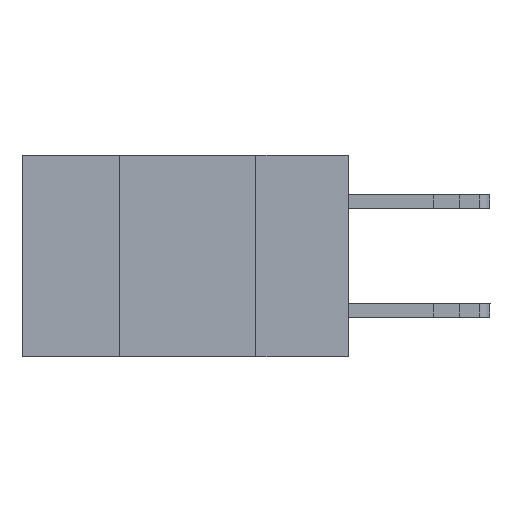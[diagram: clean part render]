
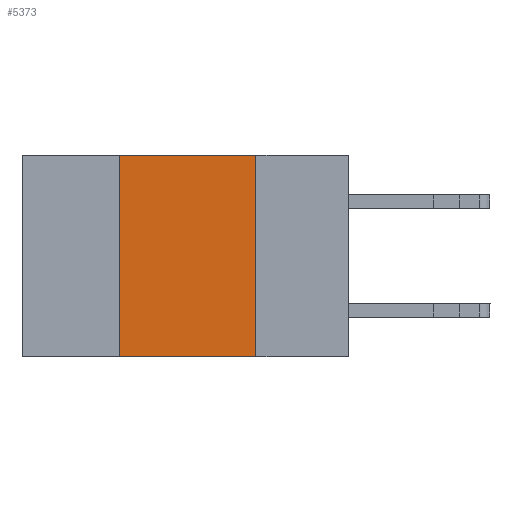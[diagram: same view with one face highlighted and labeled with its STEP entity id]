
A CAD part, left-side view. The second image highlights one B-rep face of the part: STEP entity #5373.
In plain terms, the highlighted planar face has unit normal (-1, 0, 0).
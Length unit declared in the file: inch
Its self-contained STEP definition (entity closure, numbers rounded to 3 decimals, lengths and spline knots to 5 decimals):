
#2670 = EDGE_CURVE ( 'NONE', #3437, #2915, #7472, .T. ) ;
#2915 = VERTEX_POINT ( 'NONE', #8823 ) ;
#3209 = ORIENTED_EDGE ( 'NONE', *, *, #4856, .T. ) ;
#3437 = VERTEX_POINT ( 'NONE', #11227 ) ;
#3912 = VECTOR ( 'NONE', #14967, 39.37008 ) ;
#4038 = CARTESIAN_POINT ( 'NONE',  ( 0., 0.42, -0.37 ) ) ;
#4104 = DIRECTION ( 'NONE',  ( 0., 0., 1. ) ) ;
#4520 = EDGE_CURVE ( 'NONE', #2915, #4859, #4880, .T. ) ;
#4856 = EDGE_CURVE ( 'NONE', #11636, #4859, #6945, .T. ) ;
#4859 = VERTEX_POINT ( 'NONE', #16360 ) ;
#4880 = LINE ( 'NONE', #6026, #14825 ) ;
#5124 = ORIENTED_EDGE ( 'NONE', *, *, #4520, .F. ) ;
#5373 = ADVANCED_FACE ( 'NONE', ( #12638 ), #12650, .F. ) ;
#5738 = AXIS2_PLACEMENT_3D ( 'NONE', #12631, #12607, #12588 ) ;
#5795 = VECTOR ( 'NONE', #4104, 39.37008 ) ;
#6026 = CARTESIAN_POINT ( 'NONE',  ( 0., 0.17, -0.37 ) ) ;
#6178 = DIRECTION ( 'NONE',  ( 0., 0., -1. ) ) ;
#6579 = EDGE_LOOP ( 'NONE', ( #5124, #12490, #15827, #3209 ) ) ;
#6945 = LINE ( 'NONE', #16425, #16744 ) ;
#7472 = LINE ( 'NONE', #11714, #3912 ) ;
#8426 = EDGE_CURVE ( 'NONE', #11636, #3437, #9322, .T. ) ;
#8823 = CARTESIAN_POINT ( 'NONE',  ( 0., 0.17, 0. ) ) ;
#9322 = LINE ( 'NONE', #4038, #5795 ) ;
#11227 = CARTESIAN_POINT ( 'NONE',  ( 0., 0.42, 0. ) ) ;
#11398 = CARTESIAN_POINT ( 'NONE',  ( 0., 0.42, -0.37 ) ) ;
#11636 = VERTEX_POINT ( 'NONE', #11398 ) ;
#11714 = CARTESIAN_POINT ( 'NONE',  ( 0., 0.6, 0. ) ) ;
#12490 = ORIENTED_EDGE ( 'NONE', *, *, #2670, .F. ) ;
#12588 = DIRECTION ( 'NONE',  ( 0., 0., -1. ) ) ;
#12607 = DIRECTION ( 'NONE',  ( 1., 0., 0. ) ) ;
#12631 = CARTESIAN_POINT ( 'NONE',  ( 0., 0.6, 0. ) ) ;
#12638 = FACE_OUTER_BOUND ( 'NONE', #6579, .T. ) ;
#12650 = PLANE ( 'NONE',  #5738 ) ;
#14825 = VECTOR ( 'NONE', #6178, 39.37008 ) ;
#14967 = DIRECTION ( 'NONE',  ( 0., -1., 0. ) ) ;
#15827 = ORIENTED_EDGE ( 'NONE', *, *, #8426, .F. ) ;
#16360 = CARTESIAN_POINT ( 'NONE',  ( 0., 0.17, -0.37 ) ) ;
#16388 = DIRECTION ( 'NONE',  ( 0., -1., 0. ) ) ;
#16425 = CARTESIAN_POINT ( 'NONE',  ( 0., 0.6, -0.37 ) ) ;
#16744 = VECTOR ( 'NONE', #16388, 39.37008 ) ;
